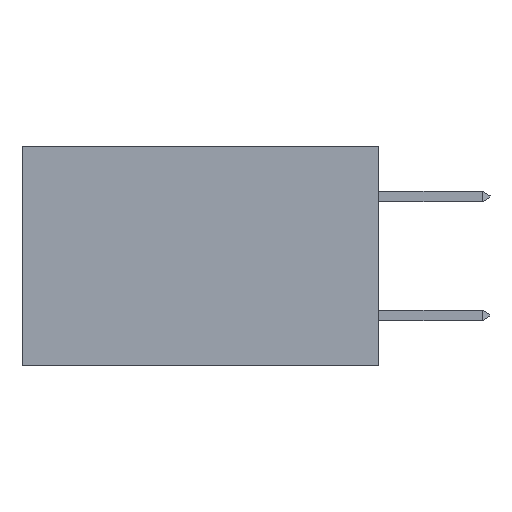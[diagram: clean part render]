
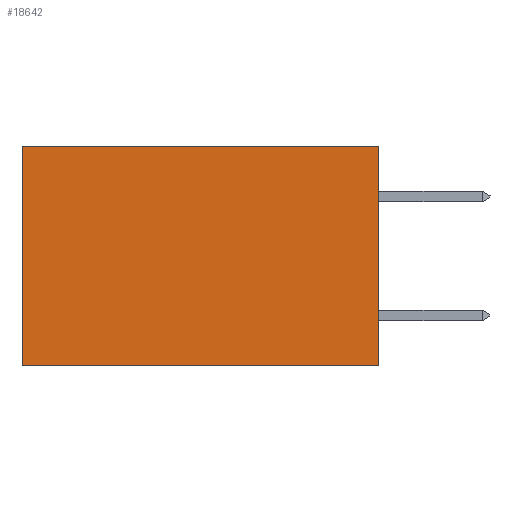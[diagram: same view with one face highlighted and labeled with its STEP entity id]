
A CAD part, left-side view. The second image highlights one B-rep face of the part: STEP entity #18642.
In plain terms, the highlighted planar face has unit normal (-1, 0, 0).
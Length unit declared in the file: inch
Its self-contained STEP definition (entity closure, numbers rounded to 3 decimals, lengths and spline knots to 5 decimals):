
#37 = CARTESIAN_POINT ( 'NONE',  ( 0.2615, 0., -0.37 ) ) ;
#1959 = VERTEX_POINT ( 'NONE', #6721 ) ;
#2292 = ORIENTED_EDGE ( 'NONE', *, *, #13402, .T. ) ;
#4508 = DIRECTION ( 'NONE',  ( 0., 0., -1. ) ) ;
#5608 = EDGE_LOOP ( 'NONE', ( #2292, #15426, #11581, #14186 ) ) ;
#6721 = CARTESIAN_POINT ( 'NONE',  ( 0.2615, 0., 0. ) ) ;
#6981 = CARTESIAN_POINT ( 'NONE',  ( 0.2615, 0.6, -0.37 ) ) ;
#10140 = CARTESIAN_POINT ( 'NONE',  ( 0.2615, 0., -0.37 ) ) ;
#10686 = VERTEX_POINT ( 'NONE', #22621 ) ;
#10708 = DIRECTION ( 'NONE',  ( 0., 1., 0. ) ) ;
#11581 = ORIENTED_EDGE ( 'NONE', *, *, #23173, .F. ) ;
#11836 = DIRECTION ( 'NONE',  ( 0., 1., 0. ) ) ;
#13402 = EDGE_CURVE ( 'NONE', #22189, #10686, #20712, .T. ) ;
#13653 = VECTOR ( 'NONE', #10708, 39.37008 ) ;
#14186 = ORIENTED_EDGE ( 'NONE', *, *, #18141, .T. ) ;
#14462 = FACE_OUTER_BOUND ( 'NONE', #5608, .T. ) ;
#14975 = CARTESIAN_POINT ( 'NONE',  ( 0.2615, 0., -0.37 ) ) ;
#15133 = CARTESIAN_POINT ( 'NONE',  ( 0.2615, 0., 0. ) ) ;
#15426 = ORIENTED_EDGE ( 'NONE', *, *, #19704, .F. ) ;
#15712 = CARTESIAN_POINT ( 'NONE',  ( 0.2615, 0.6, 0. ) ) ;
#15759 = CARTESIAN_POINT ( 'NONE',  ( 0.2615, 0., -0.37 ) ) ;
#15885 = LINE ( 'NONE', #10140, #24868 ) ;
#16279 = DIRECTION ( 'NONE',  ( 0., 0., -1. ) ) ;
#16672 = DIRECTION ( 'NONE',  ( 0., 0., -1. ) ) ;
#17990 = LINE ( 'NONE', #37, #22892 ) ;
#18141 = EDGE_CURVE ( 'NONE', #1959, #22189, #24960, .T. ) ;
#18642 = ADVANCED_FACE ( 'NONE', ( #14462 ), #24929, .F. ) ;
#19704 = EDGE_CURVE ( 'NONE', #19724, #10686, #17990, .T. ) ;
#19724 = VERTEX_POINT ( 'NONE', #15759 ) ;
#20712 = LINE ( 'NONE', #6981, #24216 ) ;
#22009 = AXIS2_PLACEMENT_3D ( 'NONE', #14975, #22695, #4508 ) ;
#22189 = VERTEX_POINT ( 'NONE', #15712 ) ;
#22621 = CARTESIAN_POINT ( 'NONE',  ( 0.2615, 0.6, -0.37 ) ) ;
#22695 = DIRECTION ( 'NONE',  ( 1., 0., 0. ) ) ;
#22892 = VECTOR ( 'NONE', #11836, 39.37008 ) ;
#23173 = EDGE_CURVE ( 'NONE', #1959, #19724, #15885, .T. ) ;
#24216 = VECTOR ( 'NONE', #16672, 39.37008 ) ;
#24868 = VECTOR ( 'NONE', #16279, 39.37008 ) ;
#24929 = PLANE ( 'NONE',  #22009 ) ;
#24960 = LINE ( 'NONE', #15133, #13653 ) ;
